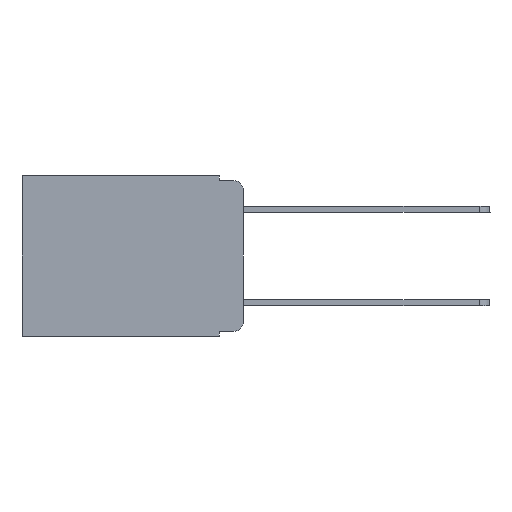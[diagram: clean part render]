
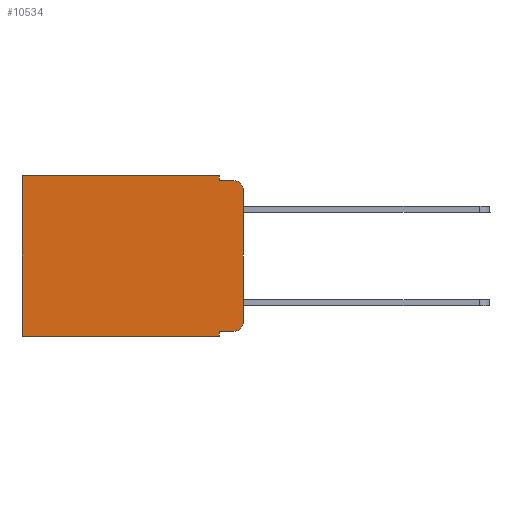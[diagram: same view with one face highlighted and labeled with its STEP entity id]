
A CAD part, left-side view. The second image highlights one B-rep face of the part: STEP entity #10534.
In plain terms, the highlighted planar face has unit normal (-1, 0, 0).
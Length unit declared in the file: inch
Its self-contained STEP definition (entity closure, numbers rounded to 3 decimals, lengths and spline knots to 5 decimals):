
#187 = VERTEX_POINT ( 'NONE', #2736 ) ;
#439 = VERTEX_POINT ( 'NONE', #3954 ) ;
#518 = ORIENTED_EDGE ( 'NONE', *, *, #10300, .F. ) ;
#703 = VERTEX_POINT ( 'NONE', #1759 ) ;
#706 = VECTOR ( 'NONE', #2812, 39.37008 ) ;
#746 = CARTESIAN_POINT ( 'NONE',  ( 0.298, 0.02, -0.313 ) ) ;
#960 = VERTEX_POINT ( 'NONE', #3337 ) ;
#1039 = CARTESIAN_POINT ( 'NONE',  ( 0.298, 0., 0. ) ) ;
#1099 = VECTOR ( 'NONE', #2186, 39.37008 ) ;
#1426 = AXIS2_PLACEMENT_3D ( 'NONE', #746, #3848, #5827 ) ;
#1563 = CARTESIAN_POINT ( 'NONE',  ( 0.298, 0.02, -0.03 ) ) ;
#1696 = EDGE_CURVE ( 'NONE', #439, #11461, #11575, .T. ) ;
#1759 = CARTESIAN_POINT ( 'NONE',  ( 0.298, 0.473, -0.343 ) ) ;
#1908 = VECTOR ( 'NONE', #10424, 39.37008 ) ;
#1966 = ORIENTED_EDGE ( 'NONE', *, *, #7392, .T. ) ;
#2051 = ORIENTED_EDGE ( 'NONE', *, *, #8052, .F. ) ;
#2113 = ORIENTED_EDGE ( 'NONE', *, *, #9440, .F. ) ;
#2186 = DIRECTION ( 'NONE',  ( 0., 1., 0. ) ) ;
#2283 = VECTOR ( 'NONE', #5022, 39.37008 ) ;
#2303 = VERTEX_POINT ( 'NONE', #9663 ) ;
#2413 = DIRECTION ( 'NONE',  ( 0., -1., 0. ) ) ;
#2574 = EDGE_CURVE ( 'NONE', #960, #703, #2837, .T. ) ;
#2679 = LINE ( 'NONE', #6549, #706 ) ;
#2736 = CARTESIAN_POINT ( 'NONE',  ( 0.298, 0.02, -0.01 ) ) ;
#2812 = DIRECTION ( 'NONE',  ( 0., 0., -1. ) ) ;
#2837 = LINE ( 'NONE', #5754, #9447 ) ;
#2841 = CARTESIAN_POINT ( 'NONE',  ( 0.298, 0.051, -0.01 ) ) ;
#2943 = CARTESIAN_POINT ( 'NONE',  ( 0.298, 0.051, -0.343 ) ) ;
#3040 = VERTEX_POINT ( 'NONE', #2943 ) ;
#3059 = CIRCLE ( 'NONE', #10107, 0.02 ) ;
#3155 = CARTESIAN_POINT ( 'NONE',  ( 0.298, 0.051, -0.333 ) ) ;
#3181 = VECTOR ( 'NONE', #11039, 39.37008 ) ;
#3337 = CARTESIAN_POINT ( 'NONE',  ( 0.298, 0.473, 0. ) ) ;
#3769 = LINE ( 'NONE', #2841, #9544 ) ;
#3848 = DIRECTION ( 'NONE',  ( -1., 0., 0. ) ) ;
#3954 = CARTESIAN_POINT ( 'NONE',  ( 0.298, 0., -0.03 ) ) ;
#4022 = VERTEX_POINT ( 'NONE', #4249 ) ;
#4249 = CARTESIAN_POINT ( 'NONE',  ( 0.298, 0.02, -0.333 ) ) ;
#4348 = CARTESIAN_POINT ( 'NONE',  ( 0.298, 0., 0. ) ) ;
#4498 = EDGE_LOOP ( 'NONE', ( #9695, #1966, #2051, #4716, #12147, #7098, #2113, #518, #9934, #9973 ) ) ;
#4716 = ORIENTED_EDGE ( 'NONE', *, *, #9338, .F. ) ;
#4980 = CARTESIAN_POINT ( 'NONE',  ( 0.298, 0., -0.343 ) ) ;
#5022 = DIRECTION ( 'NONE',  ( 0., 0., -1. ) ) ;
#5128 = DIRECTION ( 'NONE',  ( 0., 0., -1. ) ) ;
#5754 = CARTESIAN_POINT ( 'NONE',  ( 0.298, 0.473, 0. ) ) ;
#5827 = DIRECTION ( 'NONE',  ( 0., 0., -1. ) ) ;
#6221 = EDGE_CURVE ( 'NONE', #2303, #4022, #8004, .T. ) ;
#6336 = DIRECTION ( 'NONE',  ( 0., 0., -1. ) ) ;
#6549 = CARTESIAN_POINT ( 'NONE',  ( 0.298, 0.051, 0. ) ) ;
#6956 = DIRECTION ( 'NONE',  ( 0., 0., -1. ) ) ;
#7098 = ORIENTED_EDGE ( 'NONE', *, *, #2574, .T. ) ;
#7392 = EDGE_CURVE ( 'NONE', #439, #187, #3059, .T. ) ;
#7448 = VERTEX_POINT ( 'NONE', #11197 ) ;
#7551 = CARTESIAN_POINT ( 'NONE',  ( 0.298, 0.051, 0. ) ) ;
#7586 = EDGE_CURVE ( 'NONE', #4022, #11461, #10735, .T. ) ;
#7858 = LINE ( 'NONE', #4980, #1099 ) ;
#8004 = LINE ( 'NONE', #3155, #8103 ) ;
#8052 = EDGE_CURVE ( 'NONE', #7448, #187, #3769, .T. ) ;
#8103 = VECTOR ( 'NONE', #2413, 39.37008 ) ;
#8161 = LINE ( 'NONE', #9213, #3181 ) ;
#8255 = DIRECTION ( 'NONE',  ( 1., 0., 0. ) ) ;
#8278 = VERTEX_POINT ( 'NONE', #8859 ) ;
#8859 = CARTESIAN_POINT ( 'NONE',  ( 0.298, 0.051, 0. ) ) ;
#9213 = CARTESIAN_POINT ( 'NONE',  ( 0.298, 0., 0. ) ) ;
#9338 = EDGE_CURVE ( 'NONE', #8278, #7448, #12353, .T. ) ;
#9374 = DIRECTION ( 'NONE',  ( -1., 0., 0. ) ) ;
#9428 = AXIS2_PLACEMENT_3D ( 'NONE', #4348, #8255, #5128 ) ;
#9440 = EDGE_CURVE ( 'NONE', #3040, #703, #7858, .T. ) ;
#9447 = VECTOR ( 'NONE', #6956, 39.37008 ) ;
#9544 = VECTOR ( 'NONE', #10293, 39.37008 ) ;
#9663 = CARTESIAN_POINT ( 'NONE',  ( 0.298, 0.051, -0.333 ) ) ;
#9695 = ORIENTED_EDGE ( 'NONE', *, *, #1696, .F. ) ;
#9934 = ORIENTED_EDGE ( 'NONE', *, *, #6221, .T. ) ;
#9973 = ORIENTED_EDGE ( 'NONE', *, *, #7586, .T. ) ;
#10107 = AXIS2_PLACEMENT_3D ( 'NONE', #1563, #9374, #6336 ) ;
#10293 = DIRECTION ( 'NONE',  ( 0., -1., 0. ) ) ;
#10300 = EDGE_CURVE ( 'NONE', #2303, #3040, #2679, .T. ) ;
#10370 = CARTESIAN_POINT ( 'NONE',  ( 0.298, 0., -0.313 ) ) ;
#10424 = DIRECTION ( 'NONE',  ( 0., 0., -1. ) ) ;
#10534 = ADVANCED_FACE ( 'NONE', ( #12114 ), #11011, .F. ) ;
#10735 = CIRCLE ( 'NONE', #1426, 0.02 ) ;
#11011 = PLANE ( 'NONE',  #9428 ) ;
#11039 = DIRECTION ( 'NONE',  ( 0., 1., 0. ) ) ;
#11197 = CARTESIAN_POINT ( 'NONE',  ( 0.298, 0.051, -0.01 ) ) ;
#11461 = VERTEX_POINT ( 'NONE', #10370 ) ;
#11575 = LINE ( 'NONE', #1039, #2283 ) ;
#12114 = FACE_OUTER_BOUND ( 'NONE', #4498, .T. ) ;
#12147 = ORIENTED_EDGE ( 'NONE', *, *, #12310, .T. ) ;
#12310 = EDGE_CURVE ( 'NONE', #8278, #960, #8161, .T. ) ;
#12353 = LINE ( 'NONE', #7551, #1908 ) ;
